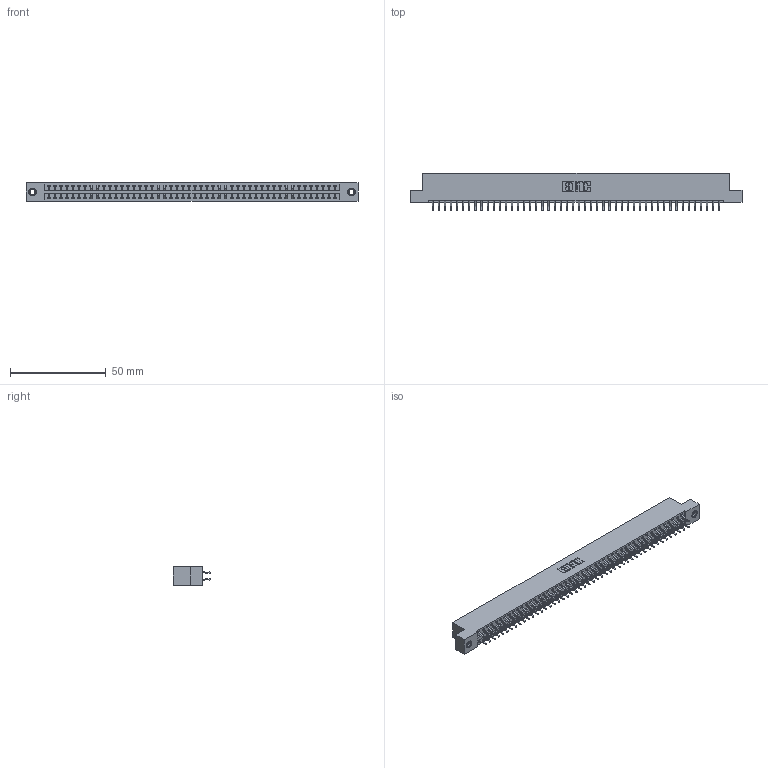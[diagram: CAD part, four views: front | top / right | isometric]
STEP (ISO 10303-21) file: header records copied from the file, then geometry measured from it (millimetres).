
FILE_DESCRIPTION (( 'STEP AP203' ), '1' );
FILE_NAME ('346-096-556-207.STEP', '2022-05-26T16:51:30', ( '' ), ( '' ), 'SwSTEP 2.0', 'SolidWorks 2020', '' );
FILE_SCHEMA (( 'CONFIG_CONTROL_DESIGN' ));
Length unit declared in the file: inch
Products named in the file (4): 345-292-001_556 Tail; 346-096-556-207; 346 Part_Flush Mounting Lugs - 0.156 Dia-TI; 345-250-001_345-250-005-103
Assembly tree (99 placements, depth 2):
  346-096-556-207
    346 Part_Flush Mounting Lugs - 0.156 Dia-TI
    345-292-001_556 Tail  x96
    345-250-001_345-250-005-103  x2
Bounding box: 172.97 x 19.57 x 9.4 mm (x, y, z)
Volume: 16896.4 mm3; surface area: 23264.1 mm2
Topology: 99 solids, 99 shells, 5750 faces, 17073 edges, 11246 vertices
Faces by surface type: plane 3852, cylinder 1882, cone 12, torus 4
Entity records: 31924 total; most frequent: CARTESIAN_POINT 5251, ORIENTED_EDGE 5166, DIRECTION 4693, EDGE_CURVE 2583, LINE 2231, VECTOR 2231, VERTEX_POINT 1716, AXIS2_PLACEMENT_3D 1231
